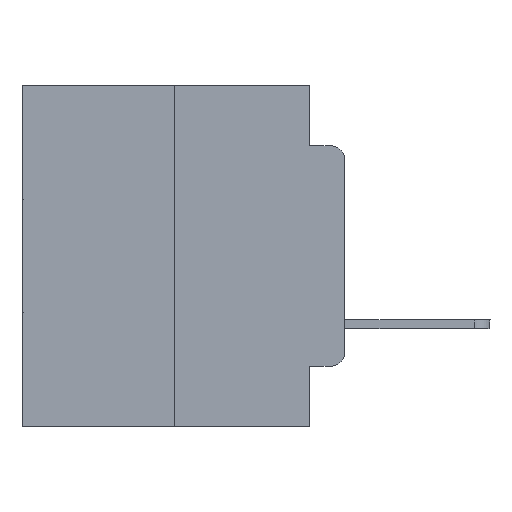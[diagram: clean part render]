
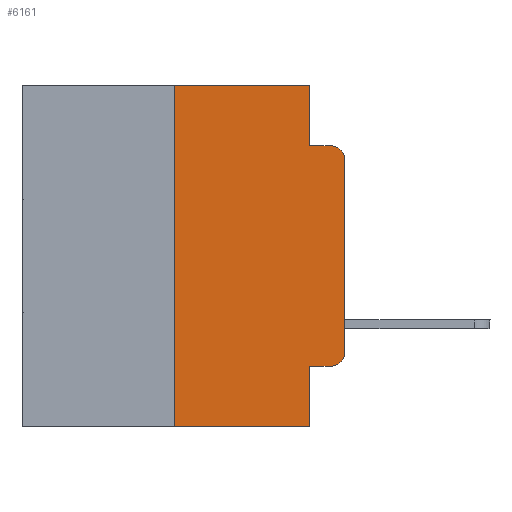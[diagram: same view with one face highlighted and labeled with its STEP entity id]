
A CAD part, left-side view. The second image highlights one B-rep face of the part: STEP entity #6161.
In plain terms, the highlighted planar face has unit normal (-1, 0, 0).
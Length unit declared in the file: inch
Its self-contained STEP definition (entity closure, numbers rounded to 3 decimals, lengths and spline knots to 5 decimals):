
#479 = DIRECTION ( 'NONE',  ( 0., 0., 1. ) ) ;
#1337 = ORIENTED_EDGE ( 'NONE', *, *, #9320, .T. ) ;
#1521 = CARTESIAN_POINT ( 'NONE',  ( 0., 0.473, 0. ) ) ;
#1556 = LINE ( 'NONE', #4012, #17990 ) ;
#2504 = LINE ( 'NONE', #20133, #18082 ) ;
#2729 = CARTESIAN_POINT ( 'NONE',  ( 0., 0., -0.1085 ) ) ;
#3369 = AXIS2_PLACEMENT_3D ( 'NONE', #1521, #10289, #3704 ) ;
#3391 = CARTESIAN_POINT ( 'NONE',  ( 0., 0.051, -0.4115 ) ) ;
#3574 = CARTESIAN_POINT ( 'NONE',  ( 0., 0.051, 0. ) ) ;
#3674 = CARTESIAN_POINT ( 'NONE',  ( 0., 0.051, -0.4115 ) ) ;
#3704 = DIRECTION ( 'NONE',  ( 0., 0., -1. ) ) ;
#3980 = FACE_OUTER_BOUND ( 'NONE', #20301, .T. ) ;
#4003 = DIRECTION ( 'NONE',  ( 0., -1., 0. ) ) ;
#4012 = CARTESIAN_POINT ( 'NONE',  ( 0., 0.473, 0. ) ) ;
#4351 = DIRECTION ( 'NONE',  ( 0., 0., 1. ) ) ;
#4374 = DIRECTION ( 'NONE',  ( -1., 0., 0. ) ) ;
#4615 = ORIENTED_EDGE ( 'NONE', *, *, #22474, .T. ) ;
#5692 = EDGE_CURVE ( 'NONE', #11984, #9870, #1556, .T. ) ;
#5994 = DIRECTION ( 'NONE',  ( 0., 0., -1. ) ) ;
#6084 = EDGE_CURVE ( 'NONE', #11578, #20758, #27498, .T. ) ;
#6161 = ADVANCED_FACE ( 'NONE', ( #3980 ), #12720, .F. ) ;
#6354 = CARTESIAN_POINT ( 'NONE',  ( 0., 0.051, -0.0885 ) ) ;
#7103 = VECTOR ( 'NONE', #10704, 39.37008 ) ;
#8007 = CIRCLE ( 'NONE', #18064, 0.02 ) ;
#8029 = EDGE_CURVE ( 'NONE', #14603, #20758, #14429, .T. ) ;
#8118 = LINE ( 'NONE', #3674, #26032 ) ;
#8302 = CARTESIAN_POINT ( 'NONE',  ( 0., 0.473, -0.5 ) ) ;
#9320 = EDGE_CURVE ( 'NONE', #25825, #21385, #8007, .T. ) ;
#9370 = EDGE_CURVE ( 'NONE', #9870, #11578, #16749, .T. ) ;
#9481 = ORIENTED_EDGE ( 'NONE', *, *, #26311, .F. ) ;
#9639 = VERTEX_POINT ( 'NONE', #3391 ) ;
#9648 = ORIENTED_EDGE ( 'NONE', *, *, #18954, .T. ) ;
#9870 = VERTEX_POINT ( 'NONE', #28266 ) ;
#10289 = DIRECTION ( 'NONE',  ( 1., 0., 0. ) ) ;
#10452 = LINE ( 'NONE', #8302, #14700 ) ;
#10540 = EDGE_CURVE ( 'NONE', #9639, #22905, #23203, .T. ) ;
#10704 = DIRECTION ( 'NONE',  ( 0., 0., -1. ) ) ;
#11549 = CARTESIAN_POINT ( 'NONE',  ( 0., 0., -0.3915 ) ) ;
#11578 = VERTEX_POINT ( 'NONE', #6354 ) ;
#11687 = AXIS2_PLACEMENT_3D ( 'NONE', #24001, #4374, #15398 ) ;
#11984 = VERTEX_POINT ( 'NONE', #22459 ) ;
#12415 = DIRECTION ( 'NONE',  ( 0., -1., 0. ) ) ;
#12505 = VECTOR ( 'NONE', #14306, 39.37008 ) ;
#12679 = CARTESIAN_POINT ( 'NONE',  ( 0., 0.25, -0.5 ) ) ;
#12720 = PLANE ( 'NONE',  #3369 ) ;
#13049 = CARTESIAN_POINT ( 'NONE',  ( 0., 0.02, -0.0885 ) ) ;
#13713 = ORIENTED_EDGE ( 'NONE', *, *, #10540, .F. ) ;
#14306 = DIRECTION ( 'NONE',  ( 0., -1., 0. ) ) ;
#14429 = CIRCLE ( 'NONE', #11687, 0.02 ) ;
#14603 = VERTEX_POINT ( 'NONE', #2729 ) ;
#14700 = VECTOR ( 'NONE', #4003, 39.37008 ) ;
#15226 = CARTESIAN_POINT ( 'NONE',  ( 0., 0., 0. ) ) ;
#15398 = DIRECTION ( 'NONE',  ( 0., 0., -1. ) ) ;
#16749 = LINE ( 'NONE', #17162, #7103 ) ;
#17162 = CARTESIAN_POINT ( 'NONE',  ( 0., 0.051, 0. ) ) ;
#17388 = ORIENTED_EDGE ( 'NONE', *, *, #27828, .T. ) ;
#17493 = CARTESIAN_POINT ( 'NONE',  ( 0., 0.02, -0.4115 ) ) ;
#17990 = VECTOR ( 'NONE', #18930, 39.37008 ) ;
#18064 = AXIS2_PLACEMENT_3D ( 'NONE', #20317, #25620, #5994 ) ;
#18082 = VECTOR ( 'NONE', #479, 39.37008 ) ;
#18270 = ORIENTED_EDGE ( 'NONE', *, *, #9370, .F. ) ;
#18930 = DIRECTION ( 'NONE',  ( 0., -1., 0. ) ) ;
#18954 = EDGE_CURVE ( 'NONE', #9639, #25825, #8118, .T. ) ;
#19053 = VECTOR ( 'NONE', #25906, 39.37008 ) ;
#19167 = ORIENTED_EDGE ( 'NONE', *, *, #5692, .F. ) ;
#19169 = CARTESIAN_POINT ( 'NONE',  ( 0., 0.051, -0.0885 ) ) ;
#19793 = ORIENTED_EDGE ( 'NONE', *, *, #6084, .F. ) ;
#19982 = ORIENTED_EDGE ( 'NONE', *, *, #8029, .T. ) ;
#20133 = CARTESIAN_POINT ( 'NONE',  ( 0., 0.25, 0. ) ) ;
#20301 = EDGE_LOOP ( 'NONE', ( #17388, #19982, #19793, #18270, #19167, #9481, #4615, #13713, #9648, #1337 ) ) ;
#20317 = CARTESIAN_POINT ( 'NONE',  ( 0., 0.02, -0.3915 ) ) ;
#20758 = VERTEX_POINT ( 'NONE', #13049 ) ;
#21155 = LINE ( 'NONE', #15226, #26843 ) ;
#21385 = VERTEX_POINT ( 'NONE', #11549 ) ;
#21426 = VERTEX_POINT ( 'NONE', #12679 ) ;
#21577 = CARTESIAN_POINT ( 'NONE',  ( 0., 0.051, -0.5 ) ) ;
#22459 = CARTESIAN_POINT ( 'NONE',  ( 0., 0.25, 0. ) ) ;
#22474 = EDGE_CURVE ( 'NONE', #21426, #22905, #10452, .T. ) ;
#22905 = VERTEX_POINT ( 'NONE', #21577 ) ;
#23203 = LINE ( 'NONE', #3574, #19053 ) ;
#24001 = CARTESIAN_POINT ( 'NONE',  ( 0., 0.02, -0.1085 ) ) ;
#25620 = DIRECTION ( 'NONE',  ( -1., 0., 0. ) ) ;
#25825 = VERTEX_POINT ( 'NONE', #17493 ) ;
#25906 = DIRECTION ( 'NONE',  ( 0., 0., -1. ) ) ;
#26032 = VECTOR ( 'NONE', #12415, 39.37008 ) ;
#26311 = EDGE_CURVE ( 'NONE', #21426, #11984, #2504, .T. ) ;
#26843 = VECTOR ( 'NONE', #4351, 39.37008 ) ;
#27498 = LINE ( 'NONE', #19169, #12505 ) ;
#27828 = EDGE_CURVE ( 'NONE', #21385, #14603, #21155, .T. ) ;
#28266 = CARTESIAN_POINT ( 'NONE',  ( 0., 0.051, 0. ) ) ;
